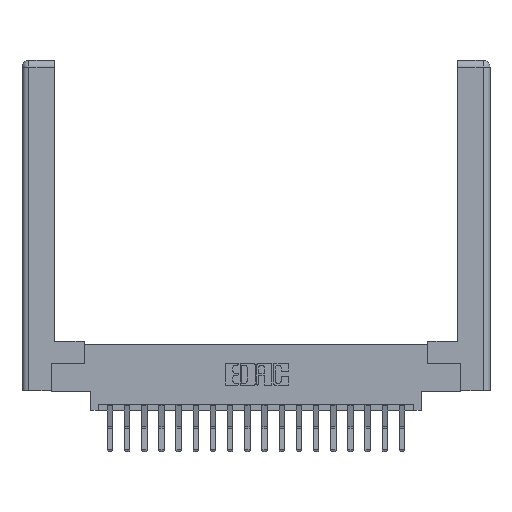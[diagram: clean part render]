
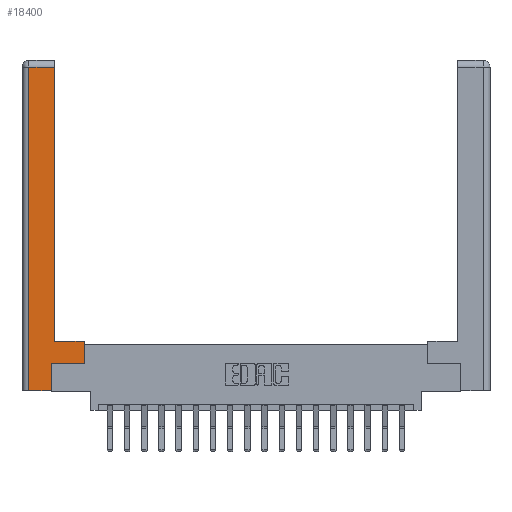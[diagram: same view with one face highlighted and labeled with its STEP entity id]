
A CAD part, top view. The second image highlights one B-rep face of the part: STEP entity #18400.
In plain terms, the highlighted planar face has unit normal (0, 0, 1).
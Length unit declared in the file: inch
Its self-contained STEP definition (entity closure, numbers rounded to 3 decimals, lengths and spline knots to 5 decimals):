
#460 = EDGE_CURVE ( 'NONE', #15174, #9615, #3572, .T. ) ;
#776 = CARTESIAN_POINT ( 'NONE',  ( 0.265, 0.245, 0. ) ) ;
#2161 = EDGE_CURVE ( 'NONE', #9615, #13378, #4457, .T. ) ;
#2332 = DIRECTION ( 'NONE',  ( 0., 1., 0. ) ) ;
#2517 = CARTESIAN_POINT ( 'NONE',  ( 0.265, 0., 0. ) ) ;
#2583 = VERTEX_POINT ( 'NONE', #7520 ) ;
#2884 = DIRECTION ( 'NONE',  ( 1., 0., 0. ) ) ;
#2964 = DIRECTION ( 'NONE',  ( 0., 0., -1. ) ) ;
#3265 = CARTESIAN_POINT ( 'NONE',  ( 0.0615, 2.94, 0. ) ) ;
#3419 = VERTEX_POINT ( 'NONE', #2517 ) ;
#3572 = LINE ( 'NONE', #16300, #9145 ) ;
#4352 = CARTESIAN_POINT ( 'NONE',  ( 0.565, 0.245, 0. ) ) ;
#4440 = PLANE ( 'NONE',  #14544 ) ;
#4457 = LINE ( 'NONE', #16005, #18214 ) ;
#5417 = VECTOR ( 'NONE', #5633, 39.37008 ) ;
#5448 = ORIENTED_EDGE ( 'NONE', *, *, #10892, .T. ) ;
#5633 = DIRECTION ( 'NONE',  ( 0., -1., 0. ) ) ;
#5753 = LINE ( 'NONE', #16493, #8408 ) ;
#5789 = EDGE_CURVE ( 'NONE', #10246, #15174, #16017, .T. ) ;
#6240 = CARTESIAN_POINT ( 'NONE',  ( 0.565, 0.45, 0. ) ) ;
#6908 = VERTEX_POINT ( 'NONE', #3265 ) ;
#7349 = LINE ( 'NONE', #19389, #5417 ) ;
#7520 = CARTESIAN_POINT ( 'NONE',  ( 0.0615, 0., 0. ) ) ;
#7745 = VECTOR ( 'NONE', #10877, 39.37008 ) ;
#8408 = VECTOR ( 'NONE', #17972, 39.37008 ) ;
#8951 = EDGE_CURVE ( 'NONE', #14971, #6908, #9645, .T. ) ;
#9145 = VECTOR ( 'NONE', #2332, 39.37008 ) ;
#9477 = ORIENTED_EDGE ( 'NONE', *, *, #460, .T. ) ;
#9615 = VERTEX_POINT ( 'NONE', #6240 ) ;
#9645 = LINE ( 'NONE', #15577, #17592 ) ;
#9835 = EDGE_LOOP ( 'NONE', ( #11586, #17663, #15215, #18403, #5448, #10607, #9477, #16504 ) ) ;
#10246 = VERTEX_POINT ( 'NONE', #776 ) ;
#10597 = CARTESIAN_POINT ( 'NONE',  ( 0.565, 0.245, 0. ) ) ;
#10607 = ORIENTED_EDGE ( 'NONE', *, *, #5789, .T. ) ;
#10877 = DIRECTION ( 'NONE',  ( 0., 1., 0. ) ) ;
#10892 = EDGE_CURVE ( 'NONE', #3419, #10246, #13512, .T. ) ;
#10901 = VECTOR ( 'NONE', #17777, 39.37008 ) ;
#11408 = EDGE_CURVE ( 'NONE', #13378, #14971, #18576, .T. ) ;
#11586 = ORIENTED_EDGE ( 'NONE', *, *, #11408, .T. ) ;
#12392 = VECTOR ( 'NONE', #2884, 39.37008 ) ;
#13378 = VERTEX_POINT ( 'NONE', #17379 ) ;
#13512 = LINE ( 'NONE', #16107, #10901 ) ;
#13566 = CARTESIAN_POINT ( 'NONE',  ( 0.295, 2.94, 0. ) ) ;
#13742 = DIRECTION ( 'NONE',  ( -1., 0., 0. ) ) ;
#14502 = DIRECTION ( 'NONE',  ( -1., 0., 0. ) ) ;
#14544 = AXIS2_PLACEMENT_3D ( 'NONE', #19879, #2964, #13742 ) ;
#14971 = VERTEX_POINT ( 'NONE', #13566 ) ;
#15174 = VERTEX_POINT ( 'NONE', #4352 ) ;
#15215 = ORIENTED_EDGE ( 'NONE', *, *, #16373, .T. ) ;
#15577 = CARTESIAN_POINT ( 'NONE',  ( 0.0615, 2.94, 0. ) ) ;
#16005 = CARTESIAN_POINT ( 'NONE',  ( 0.295, 0.45, 0. ) ) ;
#16017 = LINE ( 'NONE', #10597, #12392 ) ;
#16107 = CARTESIAN_POINT ( 'NONE',  ( 0.265, 0.245, 0. ) ) ;
#16300 = CARTESIAN_POINT ( 'NONE',  ( 0.565, 0.45, 0. ) ) ;
#16373 = EDGE_CURVE ( 'NONE', #6908, #2583, #7349, .T. ) ;
#16493 = CARTESIAN_POINT ( 'NONE',  ( 0.265, 0., 0. ) ) ;
#16504 = ORIENTED_EDGE ( 'NONE', *, *, #2161, .T. ) ;
#17226 = CARTESIAN_POINT ( 'NONE',  ( 0.295, 3., 0. ) ) ;
#17379 = CARTESIAN_POINT ( 'NONE',  ( 0.295, 0.45, 0. ) ) ;
#17592 = VECTOR ( 'NONE', #18695, 39.37008 ) ;
#17663 = ORIENTED_EDGE ( 'NONE', *, *, #8951, .T. ) ;
#17777 = DIRECTION ( 'NONE',  ( 0., 1., 0. ) ) ;
#17972 = DIRECTION ( 'NONE',  ( 1., 0., 0. ) ) ;
#18093 = FACE_OUTER_BOUND ( 'NONE', #9835, .T. ) ;
#18214 = VECTOR ( 'NONE', #14502, 39.37008 ) ;
#18400 = ADVANCED_FACE ( 'NONE', ( #18093 ), #4440, .F. ) ;
#18403 = ORIENTED_EDGE ( 'NONE', *, *, #19883, .T. ) ;
#18576 = LINE ( 'NONE', #17226, #7745 ) ;
#18695 = DIRECTION ( 'NONE',  ( -1., 0., 0. ) ) ;
#19389 = CARTESIAN_POINT ( 'NONE',  ( 0.0615, 0., 0. ) ) ;
#19879 = CARTESIAN_POINT ( 'NONE',  ( 0., 0., 0. ) ) ;
#19883 = EDGE_CURVE ( 'NONE', #2583, #3419, #5753, .T. ) ;
